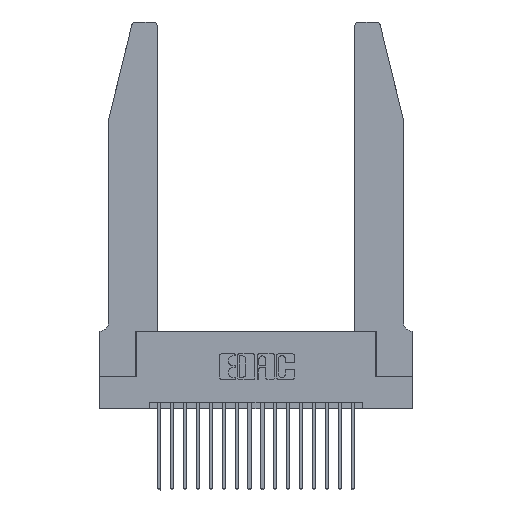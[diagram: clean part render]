
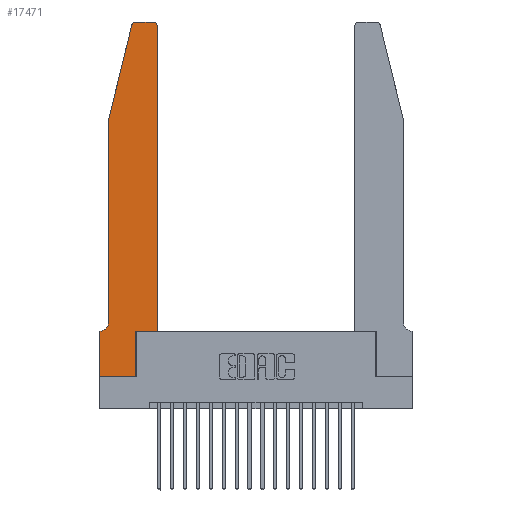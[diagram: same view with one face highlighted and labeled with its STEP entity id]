
A CAD part, top view. The second image highlights one B-rep face of the part: STEP entity #17471.
In plain terms, the highlighted planar face has unit normal (0, 0, 1).
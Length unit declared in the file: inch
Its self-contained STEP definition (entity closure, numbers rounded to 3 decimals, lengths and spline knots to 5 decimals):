
#64 = VERTEX_POINT ( 'NONE', #7960 ) ;
#279 = CARTESIAN_POINT ( 'NONE',  ( 0.2865, 0.35, 0.37 ) ) ;
#352 = CIRCLE ( 'NONE', #9258, 0.07 ) ;
#360 = DIRECTION ( 'NONE',  ( 0., -1., 0. ) ) ;
#1333 = CARTESIAN_POINT ( 'NONE',  ( 0.4505, 0.35, 0.37 ) ) ;
#1735 = ORIENTED_EDGE ( 'NONE', *, *, #11384, .T. ) ;
#1935 = DIRECTION ( 'NONE',  ( 0., 0., -1. ) ) ;
#3011 = CARTESIAN_POINT ( 'NONE',  ( 0., 0.35, 0.37 ) ) ;
#3084 = VECTOR ( 'NONE', #20598, 39.37008 ) ;
#3202 = ORIENTED_EDGE ( 'NONE', *, *, #5839, .T. ) ;
#3212 = ORIENTED_EDGE ( 'NONE', *, *, #13200, .T. ) ;
#3404 = DIRECTION ( 'NONE',  ( 0., 0., 1. ) ) ;
#3498 = ORIENTED_EDGE ( 'NONE', *, *, #19611, .T. ) ;
#3538 = CARTESIAN_POINT ( 'NONE',  ( 0.4505, 2.72, 0.37 ) ) ;
#3550 = DIRECTION ( 'NONE',  ( -0.239, -0.971, 0. ) ) ;
#3730 = VECTOR ( 'NONE', #10576, 39.37008 ) ;
#3854 = AXIS2_PLACEMENT_3D ( 'NONE', #7998, #9614, #18107 ) ;
#4057 = FACE_OUTER_BOUND ( 'NONE', #20020, .T. ) ;
#4201 = VECTOR ( 'NONE', #3550, 39.37008 ) ;
#4951 = ORIENTED_EDGE ( 'NONE', *, *, #18474, .T. ) ;
#5338 = EDGE_CURVE ( 'NONE', #14607, #15970, #11926, .T. ) ;
#5430 = DIRECTION ( 'NONE',  ( 0., 1., 0. ) ) ;
#5501 = CARTESIAN_POINT ( 'NONE',  ( 0.0755, 2., 0.37 ) ) ;
#5539 = VECTOR ( 'NONE', #9935, 39.37008 ) ;
#5839 = EDGE_CURVE ( 'NONE', #16080, #9144, #352, .T. ) ;
#6151 = CARTESIAN_POINT ( 'NONE',  ( 0.4505, 0.35, 0.37 ) ) ;
#6712 = ORIENTED_EDGE ( 'NONE', *, *, #10323, .T. ) ;
#7049 = CARTESIAN_POINT ( 'NONE',  ( 0.0055, 0.35, 0.37 ) ) ;
#7074 = LINE ( 'NONE', #8134, #5539 ) ;
#7138 = CARTESIAN_POINT ( 'NONE',  ( 0.4505, 0.35, 0.37 ) ) ;
#7530 = EDGE_CURVE ( 'NONE', #13678, #10316, #10881, .T. ) ;
#7557 = CARTESIAN_POINT ( 'NONE',  ( 0., 0., 0.37 ) ) ;
#7885 = CARTESIAN_POINT ( 'NONE',  ( 0., 0., 0.37 ) ) ;
#7960 = CARTESIAN_POINT ( 'NONE',  ( 0.2865, 0., 0.37 ) ) ;
#7998 = CARTESIAN_POINT ( 'NONE',  ( 0.284, 2.72, 0.37 ) ) ;
#8134 = CARTESIAN_POINT ( 'NONE',  ( 0.2605, 2.75, 0.37 ) ) ;
#9144 = VERTEX_POINT ( 'NONE', #7049 ) ;
#9151 = DIRECTION ( 'NONE',  ( -1., 0., 0. ) ) ;
#9258 = AXIS2_PLACEMENT_3D ( 'NONE', #9962, #1935, #11708 ) ;
#9563 = VECTOR ( 'NONE', #9151, 39.37008 ) ;
#9614 = DIRECTION ( 'NONE',  ( 0., 0., 1. ) ) ;
#9808 = CARTESIAN_POINT ( 'NONE',  ( 0.0755, 2., 0.37 ) ) ;
#9873 = DIRECTION ( 'NONE',  ( 1., 0., 0. ) ) ;
#9935 = DIRECTION ( 'NONE',  ( -1., 0., 0. ) ) ;
#9962 = CARTESIAN_POINT ( 'NONE',  ( 0.0055, 0.42, 0.37 ) ) ;
#10316 = VERTEX_POINT ( 'NONE', #3538 ) ;
#10323 = EDGE_CURVE ( 'NONE', #64, #19534, #16633, .T. ) ;
#10348 = LINE ( 'NONE', #6151, #3084 ) ;
#10576 = DIRECTION ( 'NONE',  ( 1., 0., 0. ) ) ;
#10637 = EDGE_CURVE ( 'NONE', #19534, #13678, #10348, .T. ) ;
#10881 = LINE ( 'NONE', #7138, #18404 ) ;
#11009 = PLANE ( 'NONE',  #15987 ) ;
#11031 = VECTOR ( 'NONE', #360, 39.37008 ) ;
#11349 = VERTEX_POINT ( 'NONE', #15912 ) ;
#11384 = EDGE_CURVE ( 'NONE', #10316, #20134, #19863, .T. ) ;
#11427 = EDGE_CURVE ( 'NONE', #20134, #14607, #7074, .T. ) ;
#11534 = DIRECTION ( 'NONE',  ( 0., 1., 0. ) ) ;
#11561 = ORIENTED_EDGE ( 'NONE', *, *, #17937, .T. ) ;
#11708 = DIRECTION ( 'NONE',  ( -1., 0., 0. ) ) ;
#11819 = CARTESIAN_POINT ( 'NONE',  ( 0.0755, 2., 0.37 ) ) ;
#11926 = CIRCLE ( 'NONE', #3854, 0.03 ) ;
#12297 = CARTESIAN_POINT ( 'NONE',  ( 0.284, 2.75, 0.37 ) ) ;
#12493 = VERTEX_POINT ( 'NONE', #7885 ) ;
#12612 = VECTOR ( 'NONE', #11534, 39.37008 ) ;
#12618 = ORIENTED_EDGE ( 'NONE', *, *, #5338, .T. ) ;
#12649 = AXIS2_PLACEMENT_3D ( 'NONE', #12873, #3404, #9873 ) ;
#12768 = LINE ( 'NONE', #7557, #3730 ) ;
#12873 = CARTESIAN_POINT ( 'NONE',  ( 0.4205, 2.72, 0.37 ) ) ;
#13200 = EDGE_CURVE ( 'NONE', #16122, #16080, #17040, .T. ) ;
#13235 = LINE ( 'NONE', #9808, #4201 ) ;
#13360 = CARTESIAN_POINT ( 'NONE',  ( 0.0755, 0.42, 0.37 ) ) ;
#13678 = VERTEX_POINT ( 'NONE', #1333 ) ;
#14162 = EDGE_CURVE ( 'NONE', #15970, #16122, #13235, .T. ) ;
#14174 = CARTESIAN_POINT ( 'NONE',  ( 0.4205, 2.75, 0.37 ) ) ;
#14607 = VERTEX_POINT ( 'NONE', #12297 ) ;
#14760 = CARTESIAN_POINT ( 'NONE',  ( 0.2865, 0.35, 0.37 ) ) ;
#15194 = ORIENTED_EDGE ( 'NONE', *, *, #7530, .T. ) ;
#15677 = DIRECTION ( 'NONE',  ( 0., -1., 0. ) ) ;
#15706 = DIRECTION ( 'NONE',  ( 0., 0., 1. ) ) ;
#15912 = CARTESIAN_POINT ( 'NONE',  ( 0., 0.35, 0.37 ) ) ;
#15970 = VERTEX_POINT ( 'NONE', #19551 ) ;
#15987 = AXIS2_PLACEMENT_3D ( 'NONE', #3011, #15706, #17404 ) ;
#16080 = VERTEX_POINT ( 'NONE', #13360 ) ;
#16122 = VERTEX_POINT ( 'NONE', #5501 ) ;
#16602 = LINE ( 'NONE', #20545, #19371 ) ;
#16620 = ORIENTED_EDGE ( 'NONE', *, *, #10637, .T. ) ;
#16633 = LINE ( 'NONE', #279, #12612 ) ;
#17040 = LINE ( 'NONE', #11819, #11031 ) ;
#17404 = DIRECTION ( 'NONE',  ( 1., 0., 0. ) ) ;
#17407 = ORIENTED_EDGE ( 'NONE', *, *, #14162, .T. ) ;
#17471 = ADVANCED_FACE ( 'NONE', ( #4057 ), #11009, .T. ) ;
#17937 = EDGE_CURVE ( 'NONE', #11349, #12493, #16602, .T. ) ;
#18107 = DIRECTION ( 'NONE',  ( 1., 0., 0. ) ) ;
#18404 = VECTOR ( 'NONE', #5430, 39.37008 ) ;
#18474 = EDGE_CURVE ( 'NONE', #9144, #11349, #20611, .T. ) ;
#18886 = CARTESIAN_POINT ( 'NONE',  ( 0.0755, 0.35, 0.37 ) ) ;
#19371 = VECTOR ( 'NONE', #15677, 39.37008 ) ;
#19534 = VERTEX_POINT ( 'NONE', #14760 ) ;
#19551 = CARTESIAN_POINT ( 'NONE',  ( 0.25487, 2.72718, 0.37 ) ) ;
#19611 = EDGE_CURVE ( 'NONE', #12493, #64, #12768, .T. ) ;
#19863 = CIRCLE ( 'NONE', #12649, 0.03 ) ;
#19954 = ORIENTED_EDGE ( 'NONE', *, *, #11427, .T. ) ;
#20020 = EDGE_LOOP ( 'NONE', ( #19954, #12618, #17407, #3212, #3202, #4951, #11561, #3498, #6712, #16620, #15194, #1735 ) ) ;
#20134 = VERTEX_POINT ( 'NONE', #14174 ) ;
#20545 = CARTESIAN_POINT ( 'NONE',  ( 0., 0., 0.37 ) ) ;
#20598 = DIRECTION ( 'NONE',  ( 1., 0., 0. ) ) ;
#20611 = LINE ( 'NONE', #18886, #9563 ) ;
